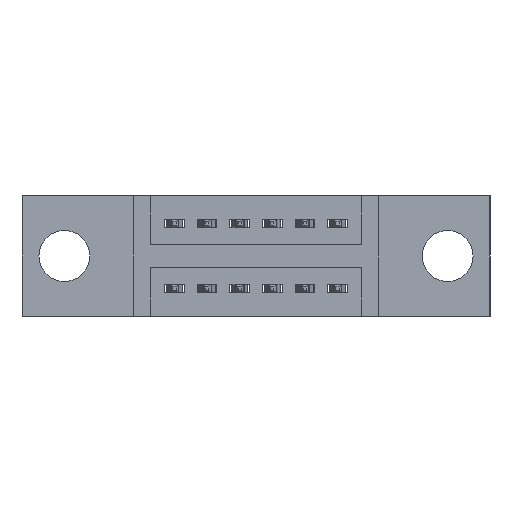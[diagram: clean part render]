
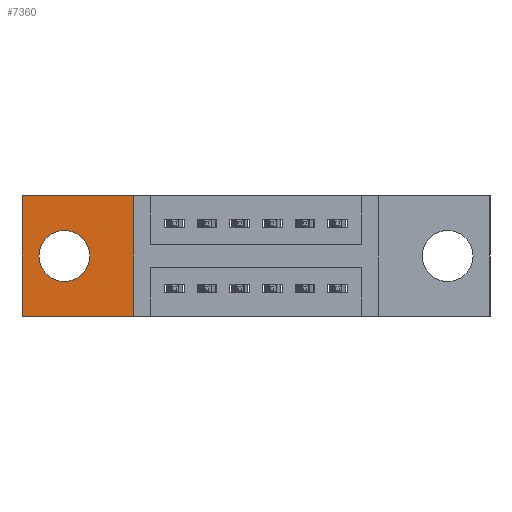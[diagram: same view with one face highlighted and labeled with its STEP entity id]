
A CAD part, front view. The second image highlights one B-rep face of the part: STEP entity #7360.
In plain terms, the highlighted planar face has unit normal (0, -1, 0).
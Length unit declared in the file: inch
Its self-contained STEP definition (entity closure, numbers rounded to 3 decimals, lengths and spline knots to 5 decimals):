
#86 = AXIS2_PLACEMENT_3D ( 'NONE', #5914, #1297, #4531 ) ;
#142 = AXIS2_PLACEMENT_3D ( 'NONE', #9216, #7778, #6800 ) ;
#182 = EDGE_CURVE ( 'NONE', #6916, #6087, #8100, .T. ) ;
#239 = ORIENTED_EDGE ( 'NONE', *, *, #182, .T. ) ;
#249 = CARTESIAN_POINT ( 'NONE',  ( 0.13, 0.11, -0.263 ) ) ;
#444 = LINE ( 'NONE', #9054, #4113 ) ;
#643 = CARTESIAN_POINT ( 'NONE',  ( 0.13, 0.11, -0.185 ) ) ;
#902 = AXIS2_PLACEMENT_3D ( 'NONE', #643, #5975, #1310 ) ;
#997 = DIRECTION ( 'NONE',  ( 1., 0., 0. ) ) ;
#1297 = DIRECTION ( 'NONE',  ( 0., -1., 0. ) ) ;
#1299 = VERTEX_POINT ( 'NONE', #9381 ) ;
#1310 = DIRECTION ( 'NONE',  ( 0., 0., -1. ) ) ;
#1383 = VERTEX_POINT ( 'NONE', #6548 ) ;
#1629 = ORIENTED_EDGE ( 'NONE', *, *, #3714, .T. ) ;
#1651 = CARTESIAN_POINT ( 'NONE',  ( 0.3425, 0.11, 0. ) ) ;
#2221 = CARTESIAN_POINT ( 'NONE',  ( 0.13, 0.11, -0.107 ) ) ;
#2796 = VERTEX_POINT ( 'NONE', #249 ) ;
#2929 = DIRECTION ( 'NONE',  ( 0., 0., -1. ) ) ;
#2962 = CARTESIAN_POINT ( 'NONE',  ( 0., 0.11, 0. ) ) ;
#3714 = EDGE_CURVE ( 'NONE', #1299, #6916, #4017, .T. ) ;
#3908 = EDGE_LOOP ( 'NONE', ( #9923, #1629, #239, #5769 ) ) ;
#4017 = LINE ( 'NONE', #8022, #4101 ) ;
#4101 = VECTOR ( 'NONE', #997, 39.37008 ) ;
#4113 = VECTOR ( 'NONE', #2929, 39.37008 ) ;
#4326 = EDGE_CURVE ( 'NONE', #1383, #1299, #444, .T. ) ;
#4531 = DIRECTION ( 'NONE',  ( 0., 0., -1. ) ) ;
#4641 = FACE_BOUND ( 'NONE', #9313, .T. ) ;
#4995 = CIRCLE ( 'NONE', #902, 0.078 ) ;
#5547 = EDGE_CURVE ( 'NONE', #2796, #7391, #4995, .T. ) ;
#5769 = ORIENTED_EDGE ( 'NONE', *, *, #10022, .T. ) ;
#5914 = CARTESIAN_POINT ( 'NONE',  ( 0.13, 0.11, -0.185 ) ) ;
#5975 = DIRECTION ( 'NONE',  ( 0., -1., 0. ) ) ;
#6020 = ORIENTED_EDGE ( 'NONE', *, *, #5547, .F. ) ;
#6022 = EDGE_CURVE ( 'NONE', #7391, #2796, #9102, .T. ) ;
#6087 = VERTEX_POINT ( 'NONE', #1651 ) ;
#6547 = CARTESIAN_POINT ( 'NONE',  ( 0.3425, 0.11, 0. ) ) ;
#6548 = CARTESIAN_POINT ( 'NONE',  ( 0., 0.11, 0. ) ) ;
#6778 = LINE ( 'NONE', #2962, #8214 ) ;
#6800 = DIRECTION ( 'NONE',  ( 0., 0., -1. ) ) ;
#6904 = FACE_OUTER_BOUND ( 'NONE', #3908, .T. ) ;
#6916 = VERTEX_POINT ( 'NONE', #9739 ) ;
#7360 = ADVANCED_FACE ( 'NONE', ( #4641, #6904 ), #8392, .T. ) ;
#7391 = VERTEX_POINT ( 'NONE', #2221 ) ;
#7778 = DIRECTION ( 'NONE',  ( 0., -1., 0. ) ) ;
#8022 = CARTESIAN_POINT ( 'NONE',  ( 0., 0.11, -0.37 ) ) ;
#8100 = LINE ( 'NONE', #6547, #8908 ) ;
#8214 = VECTOR ( 'NONE', #8313, 39.37008 ) ;
#8313 = DIRECTION ( 'NONE',  ( -1., 0., 0. ) ) ;
#8392 = PLANE ( 'NONE',  #142 ) ;
#8908 = VECTOR ( 'NONE', #9684, 39.37008 ) ;
#9054 = CARTESIAN_POINT ( 'NONE',  ( 0., 0.11, 0. ) ) ;
#9057 = ORIENTED_EDGE ( 'NONE', *, *, #6022, .F. ) ;
#9102 = CIRCLE ( 'NONE', #86, 0.078 ) ;
#9216 = CARTESIAN_POINT ( 'NONE',  ( 0., 0.11, -0.37 ) ) ;
#9313 = EDGE_LOOP ( 'NONE', ( #9057, #6020 ) ) ;
#9381 = CARTESIAN_POINT ( 'NONE',  ( 0., 0.11, -0.37 ) ) ;
#9684 = DIRECTION ( 'NONE',  ( 0., 0., 1. ) ) ;
#9739 = CARTESIAN_POINT ( 'NONE',  ( 0.3425, 0.11, -0.37 ) ) ;
#9923 = ORIENTED_EDGE ( 'NONE', *, *, #4326, .T. ) ;
#10022 = EDGE_CURVE ( 'NONE', #6087, #1383, #6778, .T. ) ;
